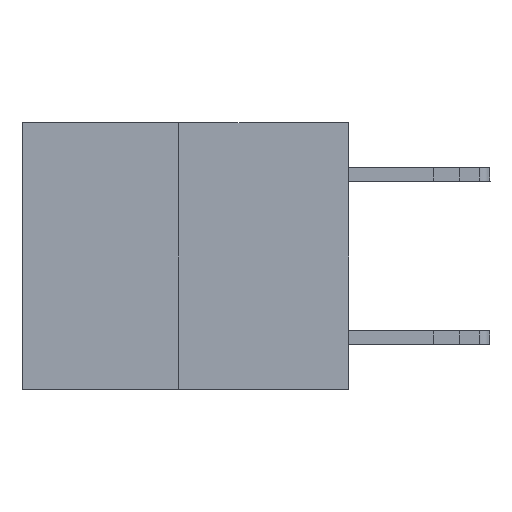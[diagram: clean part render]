
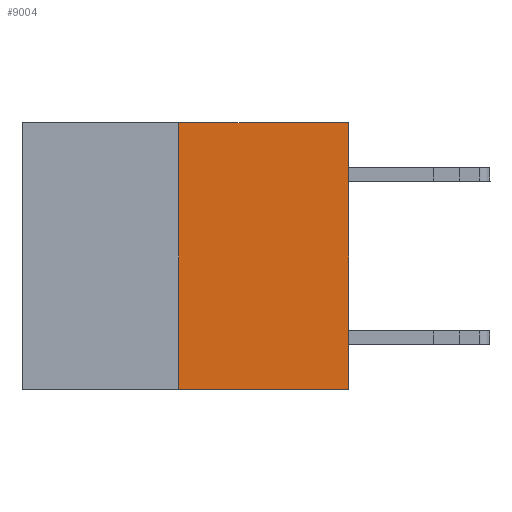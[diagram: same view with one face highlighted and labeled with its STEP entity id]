
A CAD part, left-side view. The second image highlights one B-rep face of the part: STEP entity #9004.
In plain terms, the highlighted planar face has unit normal (-1, 0, 0).
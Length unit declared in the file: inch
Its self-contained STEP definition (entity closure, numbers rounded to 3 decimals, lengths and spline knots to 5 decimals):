
#105 = LINE ( 'NONE', #5495, #17611 ) ;
#2966 = PLANE ( 'NONE',  #18207 ) ;
#3425 = FACE_OUTER_BOUND ( 'NONE', #25903, .T. ) ;
#4231 = VECTOR ( 'NONE', #14073, 39.37008 ) ;
#5276 = DIRECTION ( 'NONE',  ( 1., 0., 0. ) ) ;
#5495 = CARTESIAN_POINT ( 'NONE',  ( 0., 0.6, -0.49 ) ) ;
#5581 = VECTOR ( 'NONE', #26489, 39.37008 ) ;
#6078 = VERTEX_POINT ( 'NONE', #21791 ) ;
#6175 = DIRECTION ( 'NONE',  ( 0., 0., 1. ) ) ;
#6397 = LINE ( 'NONE', #9268, #4231 ) ;
#6992 = ORIENTED_EDGE ( 'NONE', *, *, #17887, .F. ) ;
#7388 = ORIENTED_EDGE ( 'NONE', *, *, #10756, .T. ) ;
#8368 = CARTESIAN_POINT ( 'NONE',  ( 0., 0., 0. ) ) ;
#9004 = ADVANCED_FACE ( 'NONE', ( #3425 ), #2966, .F. ) ;
#9268 = CARTESIAN_POINT ( 'NONE',  ( 0., 0.312, -0.49 ) ) ;
#10530 = CARTESIAN_POINT ( 'NONE',  ( 0., 0., 0. ) ) ;
#10672 = EDGE_CURVE ( 'NONE', #28112, #25559, #105, .T. ) ;
#10756 = EDGE_CURVE ( 'NONE', #25559, #11313, #14781, .T. ) ;
#11313 = VERTEX_POINT ( 'NONE', #10530 ) ;
#12438 = CARTESIAN_POINT ( 'NONE',  ( 0., 0.312, -0.49 ) ) ;
#12448 = CARTESIAN_POINT ( 'NONE',  ( 0., 0.6, 0. ) ) ;
#12576 = CARTESIAN_POINT ( 'NONE',  ( 0., 0., -0.49 ) ) ;
#14073 = DIRECTION ( 'NONE',  ( 0., 0., 1. ) ) ;
#14781 = LINE ( 'NONE', #8368, #19447 ) ;
#17611 = VECTOR ( 'NONE', #21521, 39.37008 ) ;
#17632 = DIRECTION ( 'NONE',  ( 0., 0., -1. ) ) ;
#17887 = EDGE_CURVE ( 'NONE', #28112, #6078, #6397, .T. ) ;
#18035 = ORIENTED_EDGE ( 'NONE', *, *, #23291, .F. ) ;
#18207 = AXIS2_PLACEMENT_3D ( 'NONE', #12448, #5276, #17632 ) ;
#19447 = VECTOR ( 'NONE', #6175, 39.37008 ) ;
#21521 = DIRECTION ( 'NONE',  ( 0., -1., 0. ) ) ;
#21791 = CARTESIAN_POINT ( 'NONE',  ( 0., 0.312, 0. ) ) ;
#21997 = CARTESIAN_POINT ( 'NONE',  ( 0., 0.6, 0. ) ) ;
#22112 = LINE ( 'NONE', #21997, #5581 ) ;
#23291 = EDGE_CURVE ( 'NONE', #6078, #11313, #22112, .T. ) ;
#25559 = VERTEX_POINT ( 'NONE', #12576 ) ;
#25903 = EDGE_LOOP ( 'NONE', ( #6992, #29026, #7388, #18035 ) ) ;
#26489 = DIRECTION ( 'NONE',  ( 0., -1., 0. ) ) ;
#28112 = VERTEX_POINT ( 'NONE', #12438 ) ;
#29026 = ORIENTED_EDGE ( 'NONE', *, *, #10672, .T. ) ;
